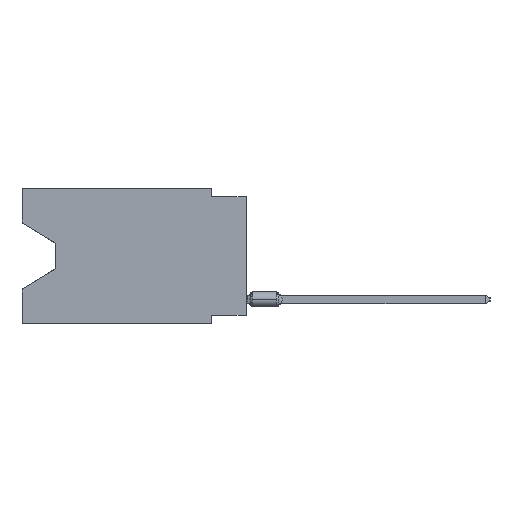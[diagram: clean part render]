
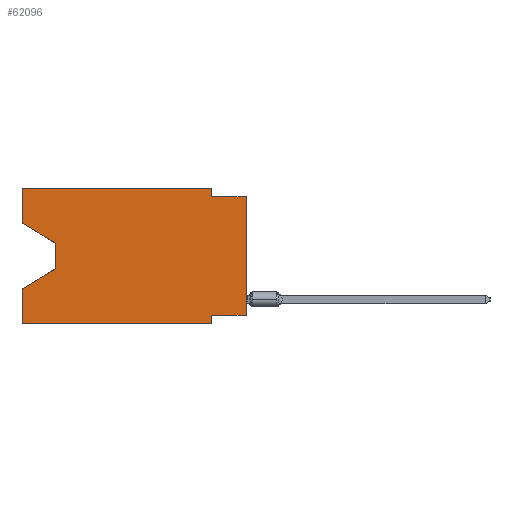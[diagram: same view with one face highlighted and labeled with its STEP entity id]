
A CAD part, left-side view. The second image highlights one B-rep face of the part: STEP entity #62096.
In plain terms, the highlighted planar face has unit normal (-1, 0, 0).
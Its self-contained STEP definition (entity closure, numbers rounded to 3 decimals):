
#609 = LINE ( 'NONE', #37588, #58767 ) ;
#883 = VECTOR ( 'NONE', #32322, 1000. ) ;
#1297 = VECTOR ( 'NONE', #20952, 1000. ) ;
#2339 = VERTEX_POINT ( 'NONE', #32062 ) ;
#2452 = EDGE_CURVE ( 'NONE', #39589, #39808, #52365, .T. ) ;
#2849 = CARTESIAN_POINT ( 'NONE',  ( 0., 2.54, -0.635 ) ) ;
#2953 = VECTOR ( 'NONE', #42981, 1000. ) ;
#4539 = CARTESIAN_POINT ( 'NONE',  ( 0., 13.97, -5.893 ) ) ;
#4542 = VERTEX_POINT ( 'NONE', #2849 ) ;
#4562 = FACE_OUTER_BOUND ( 'NONE', #18912, .T. ) ;
#4963 = EDGE_CURVE ( 'NONE', #16864, #56383, #19741, .T. ) ;
#5043 = VECTOR ( 'NONE', #52383, 1000. ) ;
#5279 = CARTESIAN_POINT ( 'NONE',  ( 0., 0., -0.635 ) ) ;
#5308 = CARTESIAN_POINT ( 'NONE',  ( 0., 13.97, -5.893 ) ) ;
#6068 = VERTEX_POINT ( 'NONE', #22559 ) ;
#7095 = EDGE_CURVE ( 'NONE', #47363, #39808, #11417, .T. ) ;
#7408 = EDGE_CURVE ( 'NONE', #15204, #6068, #31715, .T. ) ;
#8208 = CARTESIAN_POINT ( 'NONE',  ( 0., 2.54, -9.906 ) ) ;
#8390 = ORIENTED_EDGE ( 'NONE', *, *, #44223, .T. ) ;
#9806 = LINE ( 'NONE', #31065, #5043 ) ;
#11417 = LINE ( 'NONE', #38623, #34520 ) ;
#12609 = CARTESIAN_POINT ( 'NONE',  ( 0., 16.383, -2.546 ) ) ;
#13502 = ORIENTED_EDGE ( 'NONE', *, *, #33336, .F. ) ;
#13555 = CARTESIAN_POINT ( 'NONE',  ( 0., 2.54, -9.271 ) ) ;
#14837 = ORIENTED_EDGE ( 'NONE', *, *, #7408, .F. ) ;
#15204 = VERTEX_POINT ( 'NONE', #12609 ) ;
#16864 = VERTEX_POINT ( 'NONE', #59792 ) ;
#17935 = EDGE_CURVE ( 'NONE', #4542, #56383, #25865, .T. ) ;
#18912 = EDGE_LOOP ( 'NONE', ( #8390, #33299, #54343, #26621, #46344, #42610, #59364, #53286, #44417, #41874, #13502, #14837 ) ) ;
#19741 = LINE ( 'NONE', #31214, #39730 ) ;
#20280 = PLANE ( 'NONE',  #60249 ) ;
#20842 = CARTESIAN_POINT ( 'NONE',  ( 0., 16.383, -7.36 ) ) ;
#20952 = DIRECTION ( 'NONE',  ( 0., -1., 0. ) ) ;
#22559 = CARTESIAN_POINT ( 'NONE',  ( 0., 16.383, 0. ) ) ;
#22586 = LINE ( 'NONE', #59577, #883 ) ;
#24225 = VECTOR ( 'NONE', #61221, 1000. ) ;
#25163 = CARTESIAN_POINT ( 'NONE',  ( 0., 16.383, -9.906 ) ) ;
#25346 = VECTOR ( 'NONE', #26543, 1000. ) ;
#25363 = EDGE_CURVE ( 'NONE', #16864, #62361, #9806, .T. ) ;
#25819 = DIRECTION ( 'NONE',  ( 0., 0.855, -0.519 ) ) ;
#25865 = LINE ( 'NONE', #5279, #25346 ) ;
#26219 = CARTESIAN_POINT ( 'NONE',  ( 0., 16.383, -2.546 ) ) ;
#26543 = DIRECTION ( 'NONE',  ( 0., -1., 0. ) ) ;
#26621 = ORIENTED_EDGE ( 'NONE', *, *, #7095, .F. ) ;
#26851 = CARTESIAN_POINT ( 'NONE',  ( 0., 16.383, -9.906 ) ) ;
#27318 = EDGE_CURVE ( 'NONE', #62361, #68743, #45892, .T. ) ;
#27383 = CARTESIAN_POINT ( 'NONE',  ( 0., 13.97, -4.013 ) ) ;
#29460 = EDGE_CURVE ( 'NONE', #33974, #4542, #609, .T. ) ;
#31065 = CARTESIAN_POINT ( 'NONE',  ( 0., 0., -9.271 ) ) ;
#31214 = CARTESIAN_POINT ( 'NONE',  ( 0., 0., 0. ) ) ;
#31681 = VECTOR ( 'NONE', #25819, 1000. ) ;
#31715 = LINE ( 'NONE', #54419, #45710 ) ;
#32062 = CARTESIAN_POINT ( 'NONE',  ( 0., 13.97, -4.013 ) ) ;
#32322 = DIRECTION ( 'NONE',  ( 0., -1., 0. ) ) ;
#33299 = ORIENTED_EDGE ( 'NONE', *, *, #47839, .T. ) ;
#33336 = EDGE_CURVE ( 'NONE', #6068, #33974, #22586, .T. ) ;
#33974 = VERTEX_POINT ( 'NONE', #49730 ) ;
#34488 = DIRECTION ( 'NONE',  ( 0., 0., 1. ) ) ;
#34520 = VECTOR ( 'NONE', #50489, 1000. ) ;
#35246 = VECTOR ( 'NONE', #64712, 1000. ) ;
#36130 = DIRECTION ( 'NONE',  ( 0., 0., 1. ) ) ;
#36254 = EDGE_CURVE ( 'NONE', #47363, #68743, #47495, .T. ) ;
#37588 = CARTESIAN_POINT ( 'NONE',  ( 0., 2.54, 0. ) ) ;
#38623 = CARTESIAN_POINT ( 'NONE',  ( 0., 16.383, 0. ) ) ;
#39589 = VERTEX_POINT ( 'NONE', #5308 ) ;
#39730 = VECTOR ( 'NONE', #36130, 1000. ) ;
#39808 = VERTEX_POINT ( 'NONE', #20842 ) ;
#41796 = CARTESIAN_POINT ( 'NONE',  ( 0., 2.54, -9.906 ) ) ;
#41874 = ORIENTED_EDGE ( 'NONE', *, *, #29460, .F. ) ;
#42610 = ORIENTED_EDGE ( 'NONE', *, *, #27318, .F. ) ;
#42981 = DIRECTION ( 'NONE',  ( 0., -0.855, -0.519 ) ) ;
#44223 = EDGE_CURVE ( 'NONE', #15204, #2339, #47865, .T. ) ;
#44417 = ORIENTED_EDGE ( 'NONE', *, *, #17935, .F. ) ;
#45710 = VECTOR ( 'NONE', #34488, 1000. ) ;
#45892 = LINE ( 'NONE', #8208, #24225 ) ;
#46141 = CARTESIAN_POINT ( 'NONE',  ( 0., 16.383, 0. ) ) ;
#46344 = ORIENTED_EDGE ( 'NONE', *, *, #36254, .T. ) ;
#47363 = VERTEX_POINT ( 'NONE', #25163 ) ;
#47495 = LINE ( 'NONE', #26851, #1297 ) ;
#47839 = EDGE_CURVE ( 'NONE', #2339, #39589, #53569, .T. ) ;
#47865 = LINE ( 'NONE', #26219, #2953 ) ;
#49730 = CARTESIAN_POINT ( 'NONE',  ( 0., 2.54, 0. ) ) ;
#50489 = DIRECTION ( 'NONE',  ( 0., 0., 1. ) ) ;
#52365 = LINE ( 'NONE', #4539, #31681 ) ;
#52383 = DIRECTION ( 'NONE',  ( 0., 1., 0. ) ) ;
#53286 = ORIENTED_EDGE ( 'NONE', *, *, #4963, .T. ) ;
#53569 = LINE ( 'NONE', #27383, #35246 ) ;
#54343 = ORIENTED_EDGE ( 'NONE', *, *, #2452, .T. ) ;
#54419 = CARTESIAN_POINT ( 'NONE',  ( 0., 16.383, 0. ) ) ;
#54700 = DIRECTION ( 'NONE',  ( 0., 0., -1. ) ) ;
#56383 = VERTEX_POINT ( 'NONE', #68037 ) ;
#58767 = VECTOR ( 'NONE', #54700, 1000. ) ;
#59364 = ORIENTED_EDGE ( 'NONE', *, *, #25363, .F. ) ;
#59577 = CARTESIAN_POINT ( 'NONE',  ( 0., 16.383, 0. ) ) ;
#59792 = CARTESIAN_POINT ( 'NONE',  ( 0., 0., -9.271 ) ) ;
#60249 = AXIS2_PLACEMENT_3D ( 'NONE', #46141, #67376, #62488 ) ;
#61221 = DIRECTION ( 'NONE',  ( 0., 0., -1. ) ) ;
#62096 = ADVANCED_FACE ( 'NONE', ( #4562 ), #20280, .F. ) ;
#62361 = VERTEX_POINT ( 'NONE', #13555 ) ;
#62488 = DIRECTION ( 'NONE',  ( 0., 0., -1. ) ) ;
#64712 = DIRECTION ( 'NONE',  ( 0., 0., -1. ) ) ;
#67376 = DIRECTION ( 'NONE',  ( 1., 0., 0. ) ) ;
#68037 = CARTESIAN_POINT ( 'NONE',  ( 0., 0., -0.635 ) ) ;
#68743 = VERTEX_POINT ( 'NONE', #41796 ) ;
